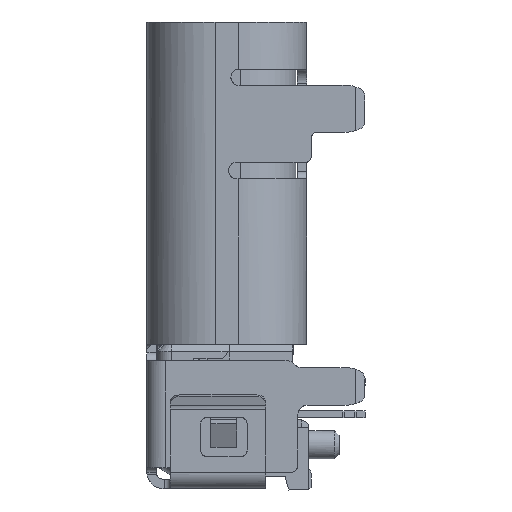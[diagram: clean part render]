
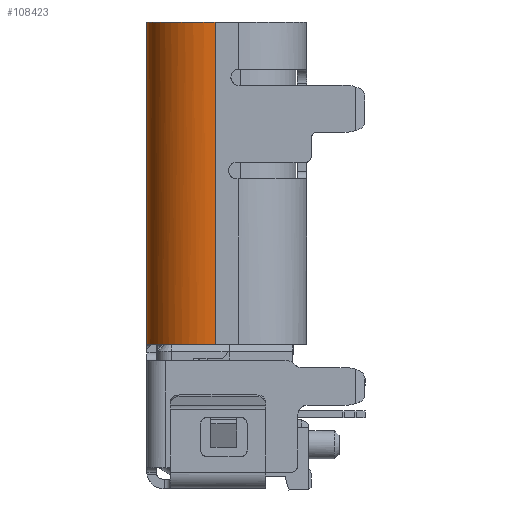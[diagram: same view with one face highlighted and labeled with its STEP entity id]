
A CAD part, left-side view. The second image highlights one B-rep face of the part: STEP entity #108423.
In plain terms, the highlighted cylindrical face has radius 1.46 mm (diameter 2.92 mm), a partial arc.
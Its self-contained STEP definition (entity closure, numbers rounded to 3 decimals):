
#1892 = CARTESIAN_POINT ( 'NONE',  ( -360.4, -0.25, -183.201 ) ) ;
#2825 = VERTEX_POINT ( 'NONE', #116197 ) ;
#6056 = CARTESIAN_POINT ( 'NONE',  ( -360.4, -0.441, -183.201 ) ) ;
#7260 = CARTESIAN_POINT ( 'NONE',  ( -360.4, -0.441, -190.111 ) ) ;
#17970 = ORIENTED_EDGE ( 'NONE', *, *, #70480, .T. ) ;
#21184 = CARTESIAN_POINT ( 'NONE',  ( -360.584, -0.985, -190.111 ) ) ;
#21615 = CARTESIAN_POINT ( 'NONE',  ( -360.4, -0.25, -190.111 ) ) ;
#25340 = CARTESIAN_POINT ( 'NONE',  ( -361.478, -1.672, -183.201 ) ) ;
#26534 = CARTESIAN_POINT ( 'NONE',  ( -361.86, -1.71, -183.201 ) ) ;
#32030 = VERTEX_POINT ( 'NONE', #63883 ) ;
#32520 = DIRECTION ( 'NONE',  ( 1., 0., 0. ) ) ;
#33738 = CARTESIAN_POINT ( 'NONE',  ( -360.584, -0.985, -183.201 ) ) ;
#36831 = VERTEX_POINT ( 'NONE', #108676 ) ;
#37683 = B_SPLINE_CURVE_WITH_KNOTS ( 'NONE', 3,
 ( #90688, #6056, #115907, #33738, #43372, #89525, #79948, #25340, #99079, #26534 ),
 .UNSPECIFIED., .F., .F.,
 ( 4, 2, 2, 2, 4 ),
 ( 0., 0.25, 0.5, 0.75, 1. ),
 .UNSPECIFIED. ) ;
#43372 = CARTESIAN_POINT ( 'NONE',  ( -360.692, -1.147, -183.201 ) ) ;
#44387 = ORIENTED_EDGE ( 'NONE', *, *, #67269, .T. ) ;
#48295 = AXIS2_PLACEMENT_3D ( 'NONE', #114709, #105070, #32520 ) ;
#49406 = CARTESIAN_POINT ( 'NONE',  ( -361.86, -1.71, -190.111 ) ) ;
#51111 = ORIENTED_EDGE ( 'NONE', *, *, #114070, .T. ) ;
#51156 = FACE_OUTER_BOUND ( 'NONE', #103656, .T. ) ;
#52354 = CARTESIAN_POINT ( 'NONE',  ( -360.4, -0.25, -190.111 ) ) ;
#55066 = CARTESIAN_POINT ( 'NONE',  ( -361.86, -1.71, -188.026 ) ) ;
#58407 = CARTESIAN_POINT ( 'NONE',  ( -361.125, -1.526, -190.111 ) ) ;
#59990 = CARTESIAN_POINT ( 'NONE',  ( -360.4, -0.25, -183.201 ) ) ;
#62901 = LINE ( 'NONE', #55066, #107907 ) ;
#63883 = CARTESIAN_POINT ( 'NONE',  ( -360.4, -0.25, -190.111 ) ) ;
#67269 = EDGE_CURVE ( 'NONE', #2825, #36831, #62901, .T. ) ;
#68517 = CARTESIAN_POINT ( 'NONE',  ( -361.478, -1.672, -190.111 ) ) ;
#70480 = EDGE_CURVE ( 'NONE', #98105, #2825, #37683, .T. ) ;
#74585 = CARTESIAN_POINT ( 'NONE',  ( -360.4, -0.25, -187.807 ) ) ;
#75789 = CARTESIAN_POINT ( 'NONE',  ( -361.669, -1.71, -190.111 ) ) ;
#76949 = CYLINDRICAL_SURFACE ( 'NONE', #48295, 1.46 ) ;
#79948 = CARTESIAN_POINT ( 'NONE',  ( -361.125, -1.526, -183.201 ) ) ;
#89525 = CARTESIAN_POINT ( 'NONE',  ( -360.963, -1.417, -183.201 ) ) ;
#90688 = CARTESIAN_POINT ( 'NONE',  ( -360.4, -0.25, -183.201 ) ) ;
#91609 = DIRECTION ( 'NONE',  ( 0., 0., -1. ) ) ;
#94960 = CARTESIAN_POINT ( 'NONE',  ( -360.963, -1.417, -190.111 ) ) ;
#94994 = EDGE_CURVE ( 'NONE', #32030, #98105, #105531, .T. ) ;
#98105 = VERTEX_POINT ( 'NONE', #1892 ) ;
#99079 = CARTESIAN_POINT ( 'NONE',  ( -361.669, -1.71, -183.201 ) ) ;
#103333 = CARTESIAN_POINT ( 'NONE',  ( -360.692, -1.147, -190.111 ) ) ;
#103656 = EDGE_LOOP ( 'NONE', ( #44387, #51111, #108556, #17970 ) ) ;
#105070 = DIRECTION ( 'NONE',  ( 0., 0., 1. ) ) ;
#105082 = CARTESIAN_POINT ( 'NONE',  ( -360.438, -0.632, -190.111 ) ) ;
#105531 = B_SPLINE_CURVE_WITH_KNOTS ( 'NONE', 3,
 ( #21615, #74585, #111139, #59990 ),
 .UNSPECIFIED., .F., .F.,
 ( 4, 4 ),
 ( 0., 1. ),
 .UNSPECIFIED. ) ;
#107907 = VECTOR ( 'NONE', #91609, 1000. ) ;
#108423 = ADVANCED_FACE ( 'NONE', ( #51156 ), #76949, .T. ) ;
#108556 = ORIENTED_EDGE ( 'NONE', *, *, #94994, .T. ) ;
#108676 = CARTESIAN_POINT ( 'NONE',  ( -361.86, -1.71, -190.111 ) ) ;
#109579 = B_SPLINE_CURVE_WITH_KNOTS ( 'NONE', 3,
 ( #49406, #75789, #68517, #58407, #94960, #103333, #21184, #105082, #7260, #52354 ),
 .UNSPECIFIED., .F., .F.,
 ( 4, 2, 2, 2, 4 ),
 ( 0., 0.25, 0.5, 0.75, 1. ),
 .UNSPECIFIED. ) ;
#111139 = CARTESIAN_POINT ( 'NONE',  ( -360.4, -0.25, -185.504 ) ) ;
#114070 = EDGE_CURVE ( 'NONE', #36831, #32030, #109579, .T. ) ;
#114709 = CARTESIAN_POINT ( 'NONE',  ( -361.86, -0.25, -190.249 ) ) ;
#115907 = CARTESIAN_POINT ( 'NONE',  ( -360.438, -0.632, -183.201 ) ) ;
#116197 = CARTESIAN_POINT ( 'NONE',  ( -361.86, -1.71, -183.201 ) ) ;
